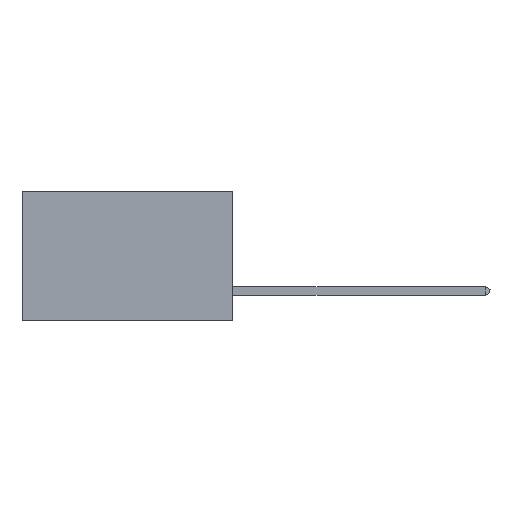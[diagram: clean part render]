
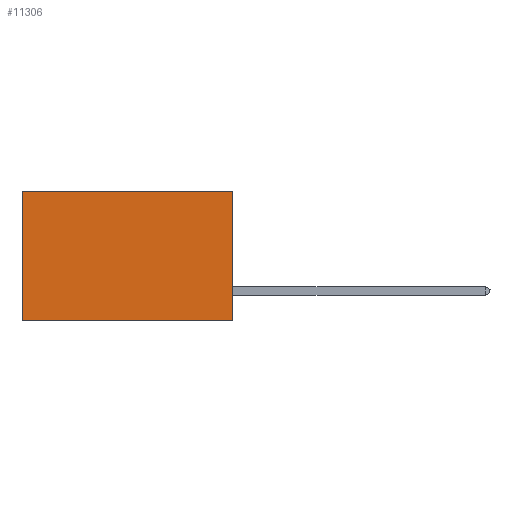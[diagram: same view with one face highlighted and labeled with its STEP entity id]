
A CAD part, left-side view. The second image highlights one B-rep face of the part: STEP entity #11306.
In plain terms, the highlighted planar face has unit normal (-1, 0, 0).
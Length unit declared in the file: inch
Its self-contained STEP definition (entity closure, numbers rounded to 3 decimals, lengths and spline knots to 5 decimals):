
#8 = CARTESIAN_POINT ( 'NONE',  ( 0.2875, 0., 0. ) ) ;
#262 = EDGE_CURVE ( 'NONE', #16449, #11669, #15480, .T. ) ;
#999 = CARTESIAN_POINT ( 'NONE',  ( 0.2875, 0., -0.37 ) ) ;
#1998 = DIRECTION ( 'NONE',  ( 0., 0., -1. ) ) ;
#2457 = VERTEX_POINT ( 'NONE', #13715 ) ;
#2869 = DIRECTION ( 'NONE',  ( 0., 1., 0. ) ) ;
#3360 = DIRECTION ( 'NONE',  ( 0., 0., -1. ) ) ;
#3446 = PLANE ( 'NONE',  #23274 ) ;
#3508 = EDGE_CURVE ( 'NONE', #2457, #20059, #7182, .T. ) ;
#4785 = CARTESIAN_POINT ( 'NONE',  ( 0.2875, 0.6, 0. ) ) ;
#5305 = LINE ( 'NONE', #24642, #14976 ) ;
#6206 = FACE_OUTER_BOUND ( 'NONE', #16599, .T. ) ;
#7024 = DIRECTION ( 'NONE',  ( 1., 0., 0. ) ) ;
#7182 = LINE ( 'NONE', #4785, #10049 ) ;
#9318 = CARTESIAN_POINT ( 'NONE',  ( 0.2875, 0., 0. ) ) ;
#10049 = VECTOR ( 'NONE', #24660, 39.37008 ) ;
#10616 = VECTOR ( 'NONE', #11425, 39.37008 ) ;
#10920 = ORIENTED_EDGE ( 'NONE', *, *, #262, .F. ) ;
#10993 = CARTESIAN_POINT ( 'NONE',  ( 0.2875, 0., -0.37 ) ) ;
#11306 = ADVANCED_FACE ( 'NONE', ( #6206 ), #3446, .F. ) ;
#11425 = DIRECTION ( 'NONE',  ( 0., 1., 0. ) ) ;
#11669 = VERTEX_POINT ( 'NONE', #999 ) ;
#12324 = ORIENTED_EDGE ( 'NONE', *, *, #12644, .F. ) ;
#12644 = EDGE_CURVE ( 'NONE', #11669, #20059, #18386, .T. ) ;
#13715 = CARTESIAN_POINT ( 'NONE',  ( 0.2875, 0.6, 0. ) ) ;
#14976 = VECTOR ( 'NONE', #2869, 39.37008 ) ;
#15480 = LINE ( 'NONE', #8, #19822 ) ;
#16449 = VERTEX_POINT ( 'NONE', #9318 ) ;
#16599 = EDGE_LOOP ( 'NONE', ( #22637, #12324, #10920, #18480 ) ) ;
#18386 = LINE ( 'NONE', #10993, #10616 ) ;
#18480 = ORIENTED_EDGE ( 'NONE', *, *, #20063, .T. ) ;
#19822 = VECTOR ( 'NONE', #1998, 39.37008 ) ;
#20059 = VERTEX_POINT ( 'NONE', #24885 ) ;
#20063 = EDGE_CURVE ( 'NONE', #16449, #2457, #5305, .T. ) ;
#22637 = ORIENTED_EDGE ( 'NONE', *, *, #3508, .T. ) ;
#23274 = AXIS2_PLACEMENT_3D ( 'NONE', #25084, #7024, #3360 ) ;
#24642 = CARTESIAN_POINT ( 'NONE',  ( 0.2875, 0., 0. ) ) ;
#24660 = DIRECTION ( 'NONE',  ( 0., 0., -1. ) ) ;
#24885 = CARTESIAN_POINT ( 'NONE',  ( 0.2875, 0.6, -0.37 ) ) ;
#25084 = CARTESIAN_POINT ( 'NONE',  ( 0.2875, 0., 0. ) ) ;
